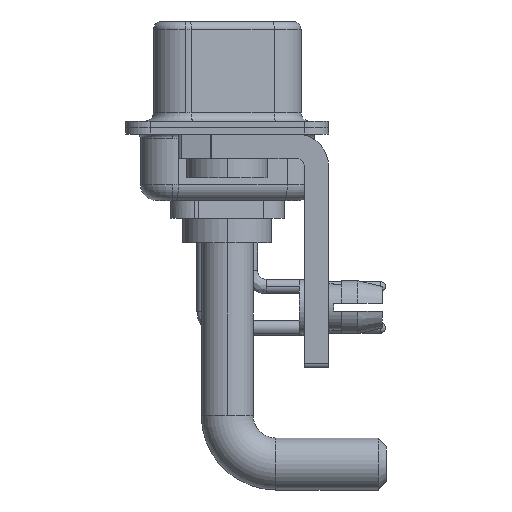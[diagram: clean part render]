
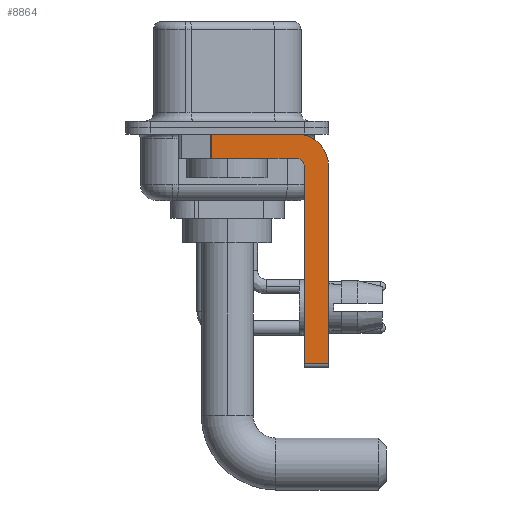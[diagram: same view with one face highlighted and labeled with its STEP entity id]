
A CAD part, left-side view. The second image highlights one B-rep face of the part: STEP entity #8864.
In plain terms, the highlighted planar face has unit normal (-1, 0, 0).
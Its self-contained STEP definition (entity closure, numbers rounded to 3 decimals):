
#378 = EDGE_CURVE ( 'NONE', #1445, #15967, #7602, .T. ) ;
#956 = LINE ( 'NONE', #27760, #4015 ) ;
#1445 = VERTEX_POINT ( 'NONE', #25564 ) ;
#1752 = CIRCLE ( 'NONE', #9791, 2. ) ;
#2981 = DIRECTION ( 'NONE',  ( 0., 1., 0. ) ) ;
#3119 = CIRCLE ( 'NONE', #12684, 0.5 ) ;
#4015 = VECTOR ( 'NONE', #27923, 1000. ) ;
#4049 = DIRECTION ( 'NONE',  ( 0., -1., 0. ) ) ;
#4133 = DIRECTION ( 'NONE',  ( 0., 0., -1. ) ) ;
#4292 = CARTESIAN_POINT ( 'NONE',  ( -2.9, 0.978, -1.9 ) ) ;
#4654 = PLANE ( 'NONE',  #28374 ) ;
#4671 = ORIENTED_EDGE ( 'NONE', *, *, #378, .F. ) ;
#4721 = EDGE_LOOP ( 'NONE', ( #17954, #15018, #26501, #4969, #4671, #13170, #9758, #17478 ) ) ;
#4969 = ORIENTED_EDGE ( 'NONE', *, *, #25526, .F. ) ;
#5472 = EDGE_CURVE ( 'NONE', #1445, #7944, #22287, .T. ) ;
#5587 = VECTOR ( 'NONE', #26313, 1000. ) ;
#6745 = VERTEX_POINT ( 'NONE', #29219 ) ;
#7319 = VERTEX_POINT ( 'NONE', #8743 ) ;
#7602 = LINE ( 'NONE', #12188, #5587 ) ;
#7944 = VERTEX_POINT ( 'NONE', #17125 ) ;
#8035 = EDGE_CURVE ( 'NONE', #18397, #7319, #29533, .T. ) ;
#8336 = CARTESIAN_POINT ( 'NONE',  ( -2.9, -4.25, -14.55 ) ) ;
#8679 = DIRECTION ( 'NONE',  ( -1., 0., 0. ) ) ;
#8743 = CARTESIAN_POINT ( 'NONE',  ( -2.9, 0.978, -1.9 ) ) ;
#8847 = LINE ( 'NONE', #4292, #30444 ) ;
#8864 = ADVANCED_FACE ( 'NONE', ( #28380 ), #4654, .F. ) ;
#9524 = CARTESIAN_POINT ( 'NONE',  ( -2.9, -4.25, -2.4 ) ) ;
#9758 = ORIENTED_EDGE ( 'NONE', *, *, #24482, .F. ) ;
#9791 = AXIS2_PLACEMENT_3D ( 'NONE', #27113, #12216, #10303 ) ;
#10303 = DIRECTION ( 'NONE',  ( 0., 0., -1. ) ) ;
#12188 = CARTESIAN_POINT ( 'NONE',  ( -2.9, -4.75, -14.8 ) ) ;
#12216 = DIRECTION ( 'NONE',  ( 1., 0., 0. ) ) ;
#12684 = AXIS2_PLACEMENT_3D ( 'NONE', #30676, #8679, #13865 ) ;
#13170 = ORIENTED_EDGE ( 'NONE', *, *, #5472, .T. ) ;
#13865 = DIRECTION ( 'NONE',  ( 0., 0., 1. ) ) ;
#13902 = VERTEX_POINT ( 'NONE', #16640 ) ;
#15018 = ORIENTED_EDGE ( 'NONE', *, *, #30341, .T. ) ;
#15784 = VECTOR ( 'NONE', #4049, 1000. ) ;
#15967 = VERTEX_POINT ( 'NONE', #19127 ) ;
#16640 = CARTESIAN_POINT ( 'NONE',  ( -2.9, -4.25, -0.4 ) ) ;
#17125 = CARTESIAN_POINT ( 'NONE',  ( -2.9, -6.25, -14.55 ) ) ;
#17478 = ORIENTED_EDGE ( 'NONE', *, *, #29676, .F. ) ;
#17745 = CARTESIAN_POINT ( 'NONE',  ( -2.9, -6.25, -2.4 ) ) ;
#17911 = DIRECTION ( 'NONE',  ( 0., -1., 0. ) ) ;
#17954 = ORIENTED_EDGE ( 'NONE', *, *, #29426, .F. ) ;
#18056 = CARTESIAN_POINT ( 'NONE',  ( -2.9, -4.25, -1.9 ) ) ;
#18397 = VERTEX_POINT ( 'NONE', #27848 ) ;
#19127 = CARTESIAN_POINT ( 'NONE',  ( -2.9, -4.75, -2.4 ) ) ;
#19260 = DIRECTION ( 'NONE',  ( 0., 0., -1. ) ) ;
#20231 = LINE ( 'NONE', #27939, #15784 ) ;
#21218 = VECTOR ( 'NONE', #17911, 1000. ) ;
#21372 = VECTOR ( 'NONE', #2981, 1000. ) ;
#21608 = DIRECTION ( 'NONE',  ( 1., 0., 0. ) ) ;
#22287 = LINE ( 'NONE', #8336, #21218 ) ;
#24482 = EDGE_CURVE ( 'NONE', #27014, #7944, #956, .T. ) ;
#25526 = EDGE_CURVE ( 'NONE', #15967, #18397, #3119, .T. ) ;
#25564 = CARTESIAN_POINT ( 'NONE',  ( -2.9, -4.75, -14.55 ) ) ;
#26313 = DIRECTION ( 'NONE',  ( 0., 0., 1. ) ) ;
#26501 = ORIENTED_EDGE ( 'NONE', *, *, #8035, .F. ) ;
#27014 = VERTEX_POINT ( 'NONE', #17745 ) ;
#27113 = CARTESIAN_POINT ( 'NONE',  ( -2.9, -4.25, -2.4 ) ) ;
#27760 = CARTESIAN_POINT ( 'NONE',  ( -2.9, -6.25, -2.4 ) ) ;
#27848 = CARTESIAN_POINT ( 'NONE',  ( -2.9, -4.25, -1.9 ) ) ;
#27923 = DIRECTION ( 'NONE',  ( 0., 0., -1. ) ) ;
#27939 = CARTESIAN_POINT ( 'NONE',  ( -2.9, 3., -0.4 ) ) ;
#28374 = AXIS2_PLACEMENT_3D ( 'NONE', #9524, #21608, #19260 ) ;
#28380 = FACE_OUTER_BOUND ( 'NONE', #4721, .T. ) ;
#29219 = CARTESIAN_POINT ( 'NONE',  ( -2.9, 0.978, -0.4 ) ) ;
#29426 = EDGE_CURVE ( 'NONE', #6745, #13902, #20231, .T. ) ;
#29533 = LINE ( 'NONE', #18056, #21372 ) ;
#29676 = EDGE_CURVE ( 'NONE', #13902, #27014, #1752, .T. ) ;
#30341 = EDGE_CURVE ( 'NONE', #6745, #7319, #8847, .T. ) ;
#30444 = VECTOR ( 'NONE', #4133, 1000. ) ;
#30676 = CARTESIAN_POINT ( 'NONE',  ( -2.9, -4.25, -2.4 ) ) ;
